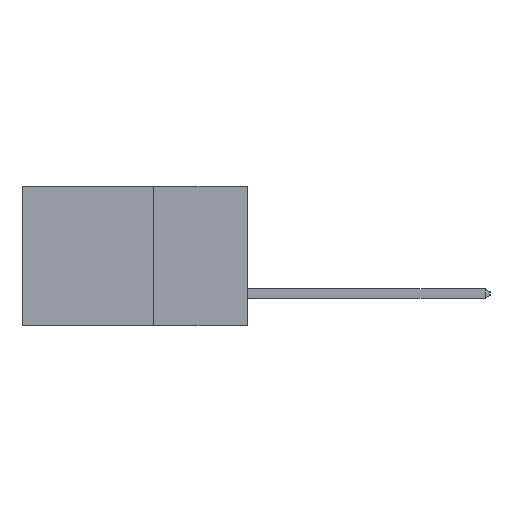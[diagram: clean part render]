
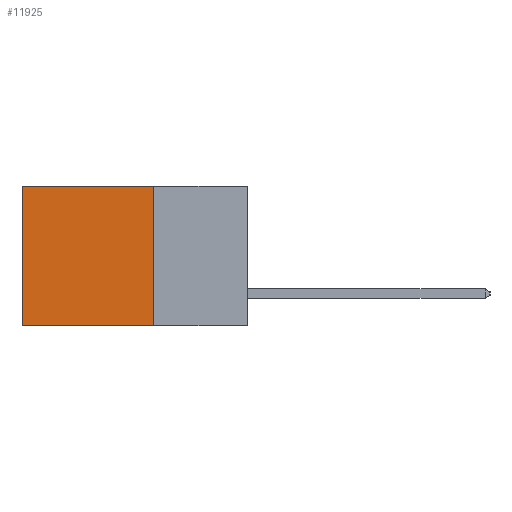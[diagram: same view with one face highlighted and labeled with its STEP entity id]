
A CAD part, left-side view. The second image highlights one B-rep face of the part: STEP entity #11925.
In plain terms, the highlighted planar face has unit normal (-1, 0, 0).
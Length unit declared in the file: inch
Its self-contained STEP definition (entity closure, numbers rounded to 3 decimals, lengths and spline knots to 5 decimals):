
#1664 = FACE_OUTER_BOUND ( 'NONE', #7480, .T. ) ;
#1799 = VERTEX_POINT ( 'NONE', #13778 ) ;
#2234 = LINE ( 'NONE', #3101, #19048 ) ;
#2475 = VERTEX_POINT ( 'NONE', #5948 ) ;
#3101 = CARTESIAN_POINT ( 'NONE',  ( 0.2615, 0.25, 0. ) ) ;
#3103 = DIRECTION ( 'NONE',  ( 0., 1., 0. ) ) ;
#3462 = PLANE ( 'NONE',  #13444 ) ;
#4063 = VERTEX_POINT ( 'NONE', #20135 ) ;
#4952 = EDGE_CURVE ( 'NONE', #4063, #2475, #2234, .T. ) ;
#5057 = VECTOR ( 'NONE', #15025, 39.37008 ) ;
#5086 = DIRECTION ( 'NONE',  ( 0., 0., -1. ) ) ;
#5251 = EDGE_CURVE ( 'NONE', #2475, #1799, #17678, .T. ) ;
#5935 = VECTOR ( 'NONE', #9320, 39.37008 ) ;
#5948 = CARTESIAN_POINT ( 'NONE',  ( 0.2615, 0.6, 0. ) ) ;
#6016 = VECTOR ( 'NONE', #7691, 39.37008 ) ;
#7480 = EDGE_LOOP ( 'NONE', ( #14016, #10624, #10641, #19841 ) ) ;
#7691 = DIRECTION ( 'NONE',  ( 0., 1., 0. ) ) ;
#7707 = CARTESIAN_POINT ( 'NONE',  ( 0.2615, 0.25, -0.37 ) ) ;
#7711 = CARTESIAN_POINT ( 'NONE',  ( 0.2615, 0.25, -0.37 ) ) ;
#9320 = DIRECTION ( 'NONE',  ( 0., 0., -1. ) ) ;
#9898 = EDGE_CURVE ( 'NONE', #14946, #1799, #10780, .T. ) ;
#10624 = ORIENTED_EDGE ( 'NONE', *, *, #9898, .F. ) ;
#10641 = ORIENTED_EDGE ( 'NONE', *, *, #19780, .F. ) ;
#10780 = LINE ( 'NONE', #7711, #6016 ) ;
#11925 = ADVANCED_FACE ( 'NONE', ( #1664 ), #3462, .F. ) ;
#13060 = CARTESIAN_POINT ( 'NONE',  ( 0.2615, 0.25, -0.37 ) ) ;
#13444 = AXIS2_PLACEMENT_3D ( 'NONE', #13060, #14656, #5086 ) ;
#13778 = CARTESIAN_POINT ( 'NONE',  ( 0.2615, 0.6, -0.37 ) ) ;
#14016 = ORIENTED_EDGE ( 'NONE', *, *, #5251, .T. ) ;
#14413 = LINE ( 'NONE', #7707, #5935 ) ;
#14656 = DIRECTION ( 'NONE',  ( 1., 0., 0. ) ) ;
#14946 = VERTEX_POINT ( 'NONE', #17620 ) ;
#15025 = DIRECTION ( 'NONE',  ( 0., 0., -1. ) ) ;
#15095 = CARTESIAN_POINT ( 'NONE',  ( 0.2615, 0.6, -0.37 ) ) ;
#17620 = CARTESIAN_POINT ( 'NONE',  ( 0.2615, 0.25, -0.37 ) ) ;
#17678 = LINE ( 'NONE', #15095, #5057 ) ;
#19048 = VECTOR ( 'NONE', #3103, 39.37008 ) ;
#19780 = EDGE_CURVE ( 'NONE', #4063, #14946, #14413, .T. ) ;
#19841 = ORIENTED_EDGE ( 'NONE', *, *, #4952, .T. ) ;
#20135 = CARTESIAN_POINT ( 'NONE',  ( 0.2615, 0.25, 0. ) ) ;
